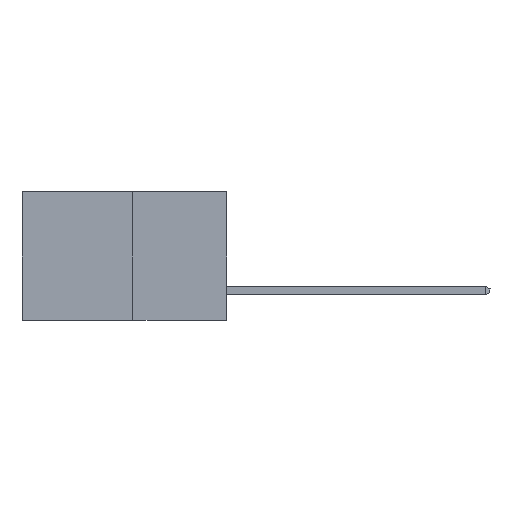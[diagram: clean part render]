
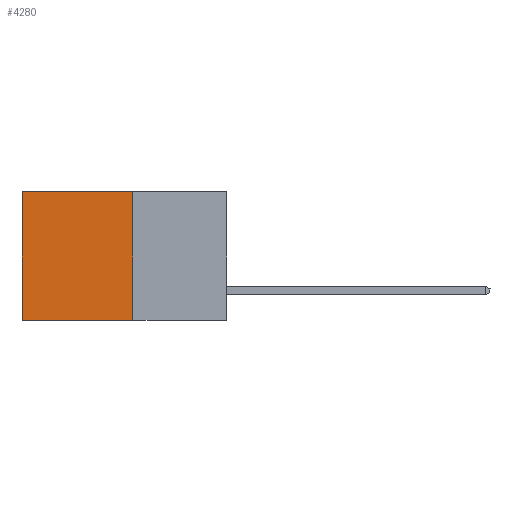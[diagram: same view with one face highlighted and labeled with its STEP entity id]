
A CAD part, left-side view. The second image highlights one B-rep face of the part: STEP entity #4280.
In plain terms, the highlighted planar face has unit normal (-1, 0, 0).
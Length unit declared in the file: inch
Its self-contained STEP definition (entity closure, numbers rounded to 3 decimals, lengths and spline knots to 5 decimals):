
#34 = LINE ( 'NONE', #12094, #7780 ) ;
#341 = AXIS2_PLACEMENT_3D ( 'NONE', #3032, #2914, #2901 ) ;
#573 = EDGE_CURVE ( 'NONE', #4032, #3542, #2186, .T. ) ;
#789 = VERTEX_POINT ( 'NONE', #7905 ) ;
#1485 = VECTOR ( 'NONE', #9726, 39.37008 ) ;
#1657 = ORIENTED_EDGE ( 'NONE', *, *, #2366, .F. ) ;
#2186 = LINE ( 'NONE', #2313, #9789 ) ;
#2205 = ORIENTED_EDGE ( 'NONE', *, *, #3166, .T. ) ;
#2313 = CARTESIAN_POINT ( 'NONE',  ( 0.277, 0.27, -0.37 ) ) ;
#2366 = EDGE_CURVE ( 'NONE', #789, #4032, #34, .T. ) ;
#2518 = CARTESIAN_POINT ( 'NONE',  ( 0.277, 0.27, -0.37 ) ) ;
#2752 = DIRECTION ( 'NONE',  ( 0., 1., 0. ) ) ;
#2901 = DIRECTION ( 'NONE',  ( 0., 0., -1. ) ) ;
#2914 = DIRECTION ( 'NONE',  ( 1., 0., 0. ) ) ;
#2990 = PLANE ( 'NONE',  #341 ) ;
#3032 = CARTESIAN_POINT ( 'NONE',  ( 0.277, 0.27, -0.37 ) ) ;
#3166 = EDGE_CURVE ( 'NONE', #6106, #3542, #4214, .T. ) ;
#3542 = VERTEX_POINT ( 'NONE', #5459 ) ;
#3575 = EDGE_CURVE ( 'NONE', #789, #6106, #9734, .T. ) ;
#4032 = VERTEX_POINT ( 'NONE', #2518 ) ;
#4214 = LINE ( 'NONE', #7678, #1485 ) ;
#4280 = ADVANCED_FACE ( 'NONE', ( #11761 ), #2990, .F. ) ;
#5459 = CARTESIAN_POINT ( 'NONE',  ( 0.277, 0.59, -0.37 ) ) ;
#5627 = CARTESIAN_POINT ( 'NONE',  ( 0.277, 0.27, 0. ) ) ;
#5957 = CARTESIAN_POINT ( 'NONE',  ( 0.277, 0.59, 0. ) ) ;
#6106 = VERTEX_POINT ( 'NONE', #5957 ) ;
#6268 = ORIENTED_EDGE ( 'NONE', *, *, #573, .F. ) ;
#6876 = DIRECTION ( 'NONE',  ( 0., 1., 0. ) ) ;
#7151 = VECTOR ( 'NONE', #6876, 39.37008 ) ;
#7312 = EDGE_LOOP ( 'NONE', ( #2205, #6268, #1657, #12762 ) ) ;
#7678 = CARTESIAN_POINT ( 'NONE',  ( 0.277, 0.59, -0.37 ) ) ;
#7780 = VECTOR ( 'NONE', #12082, 39.37008 ) ;
#7905 = CARTESIAN_POINT ( 'NONE',  ( 0.277, 0.27, 0. ) ) ;
#9726 = DIRECTION ( 'NONE',  ( 0., 0., -1. ) ) ;
#9734 = LINE ( 'NONE', #5627, #7151 ) ;
#9789 = VECTOR ( 'NONE', #2752, 39.37008 ) ;
#11761 = FACE_OUTER_BOUND ( 'NONE', #7312, .T. ) ;
#12082 = DIRECTION ( 'NONE',  ( 0., 0., -1. ) ) ;
#12094 = CARTESIAN_POINT ( 'NONE',  ( 0.277, 0.27, -0.37 ) ) ;
#12762 = ORIENTED_EDGE ( 'NONE', *, *, #3575, .T. ) ;
